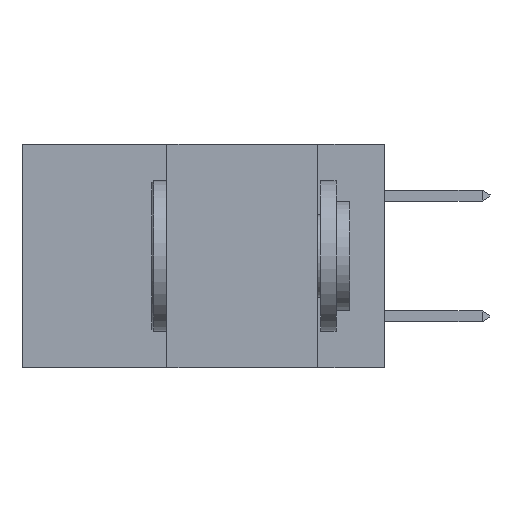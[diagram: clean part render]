
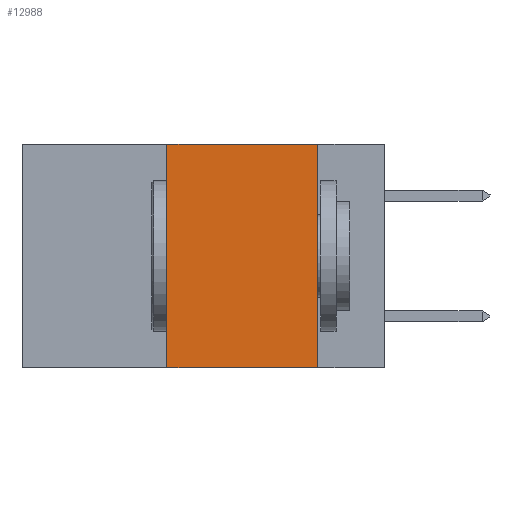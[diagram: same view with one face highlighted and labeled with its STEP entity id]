
A CAD part, left-side view. The second image highlights one B-rep face of the part: STEP entity #12988.
In plain terms, the highlighted planar face has unit normal (-1, 0, 0).
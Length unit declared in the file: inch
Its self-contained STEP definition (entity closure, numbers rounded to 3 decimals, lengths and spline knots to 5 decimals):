
#2035 = CARTESIAN_POINT ( 'NONE',  ( 0., 0.36, -0.37 ) ) ;
#2127 = CARTESIAN_POINT ( 'NONE',  ( 0., 0.6, -0.37 ) ) ;
#2533 = PLANE ( 'NONE',  #12905 ) ;
#3101 = DIRECTION ( 'NONE',  ( 0., 0., 1. ) ) ;
#3634 = LINE ( 'NONE', #15760, #6583 ) ;
#4305 = DIRECTION ( 'NONE',  ( 0., -1., 0. ) ) ;
#6583 = VECTOR ( 'NONE', #24364, 39.37008 ) ;
#7193 = VERTEX_POINT ( 'NONE', #11186 ) ;
#7735 = VECTOR ( 'NONE', #8535, 39.37008 ) ;
#8263 = EDGE_CURVE ( 'NONE', #26452, #15569, #23464, .T. ) ;
#8315 = FACE_OUTER_BOUND ( 'NONE', #16290, .T. ) ;
#8535 = DIRECTION ( 'NONE',  ( 0., 0., -1. ) ) ;
#10573 = ORIENTED_EDGE ( 'NONE', *, *, #21159, .T. ) ;
#10608 = CARTESIAN_POINT ( 'NONE',  ( 0., 0.11, 0. ) ) ;
#11186 = CARTESIAN_POINT ( 'NONE',  ( 0., 0.11, -0.37 ) ) ;
#12436 = VERTEX_POINT ( 'NONE', #15401 ) ;
#12522 = VECTOR ( 'NONE', #3101, 39.37008 ) ;
#12905 = AXIS2_PLACEMENT_3D ( 'NONE', #18883, #19150, #23280 ) ;
#12988 = ADVANCED_FACE ( 'NONE', ( #8315 ), #2533, .F. ) ;
#15022 = VECTOR ( 'NONE', #4305, 39.37008 ) ;
#15401 = CARTESIAN_POINT ( 'NONE',  ( 0., 0.11, 0. ) ) ;
#15569 = VERTEX_POINT ( 'NONE', #24899 ) ;
#15760 = CARTESIAN_POINT ( 'NONE',  ( 0., 0.6, 0. ) ) ;
#16290 = EDGE_LOOP ( 'NONE', ( #19357, #25161, #24383, #10573 ) ) ;
#18666 = EDGE_CURVE ( 'NONE', #12436, #7193, #18688, .T. ) ;
#18688 = LINE ( 'NONE', #10608, #7735 ) ;
#18883 = CARTESIAN_POINT ( 'NONE',  ( 0., 0.6, 0. ) ) ;
#19150 = DIRECTION ( 'NONE',  ( 1., 0., 0. ) ) ;
#19357 = ORIENTED_EDGE ( 'NONE', *, *, #18666, .F. ) ;
#20483 = LINE ( 'NONE', #2127, #15022 ) ;
#21159 = EDGE_CURVE ( 'NONE', #26452, #7193, #20483, .T. ) ;
#23280 = DIRECTION ( 'NONE',  ( 0., 0., -1. ) ) ;
#23464 = LINE ( 'NONE', #23663, #12522 ) ;
#23663 = CARTESIAN_POINT ( 'NONE',  ( 0., 0.36, 0. ) ) ;
#24364 = DIRECTION ( 'NONE',  ( 0., -1., 0. ) ) ;
#24383 = ORIENTED_EDGE ( 'NONE', *, *, #8263, .F. ) ;
#24417 = EDGE_CURVE ( 'NONE', #15569, #12436, #3634, .T. ) ;
#24899 = CARTESIAN_POINT ( 'NONE',  ( 0., 0.36, 0. ) ) ;
#25161 = ORIENTED_EDGE ( 'NONE', *, *, #24417, .F. ) ;
#26452 = VERTEX_POINT ( 'NONE', #2035 ) ;
